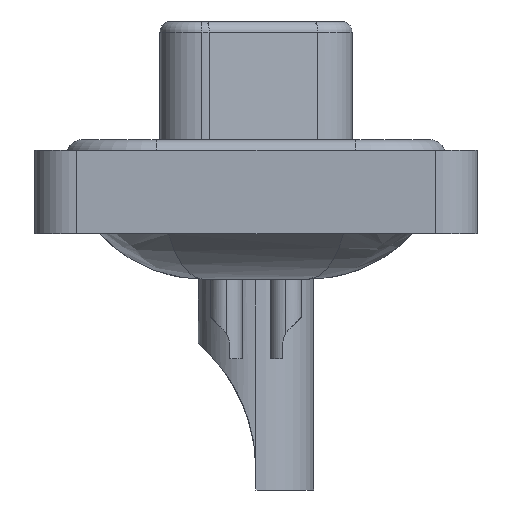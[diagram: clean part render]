
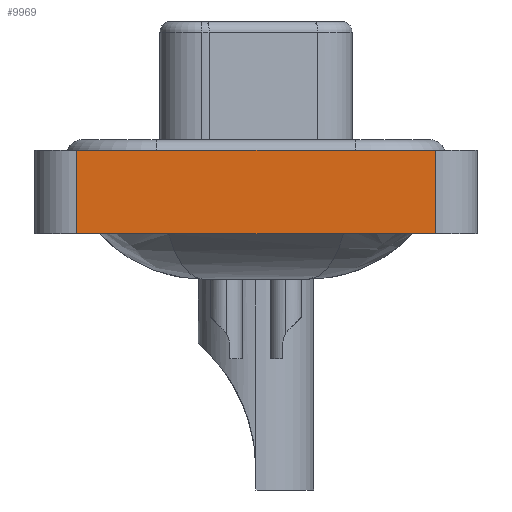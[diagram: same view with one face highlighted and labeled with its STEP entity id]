
A CAD part, left-side view. The second image highlights one B-rep face of the part: STEP entity #9969.
In plain terms, the highlighted planar face has unit normal (-1, 0, 0).
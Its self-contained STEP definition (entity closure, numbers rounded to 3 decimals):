
#1512 = CARTESIAN_POINT ( 'NONE',  ( -7.35, -8.55, -3.6 ) ) ;
#1680 = EDGE_CURVE ( 'NONE', #20873, #17307, #14497, .T. ) ;
#1867 = DIRECTION ( 'NONE',  ( -1., 0., 0. ) ) ;
#1883 = LINE ( 'NONE', #1512, #20298 ) ;
#2558 = ORIENTED_EDGE ( 'NONE', *, *, #10255, .T. ) ;
#2963 = CARTESIAN_POINT ( 'NONE',  ( -7.35, -8.55, -3.6 ) ) ;
#3530 = VECTOR ( 'NONE', #10609, 1000. ) ;
#4002 = PLANE ( 'NONE',  #15526 ) ;
#4175 = VECTOR ( 'NONE', #16267, 1000. ) ;
#6717 = LINE ( 'NONE', #2963, #3530 ) ;
#6854 = DIRECTION ( 'NONE',  ( 0., -1., 0. ) ) ;
#7087 = EDGE_LOOP ( 'NONE', ( #19540, #9354, #21882, #2558 ) ) ;
#7656 = FACE_OUTER_BOUND ( 'NONE', #7087, .T. ) ;
#8632 = CARTESIAN_POINT ( 'NONE',  ( -7.35, 8.55, -3.6 ) ) ;
#8835 = CARTESIAN_POINT ( 'NONE',  ( -7.35, -8.55, -3.6 ) ) ;
#8847 = CARTESIAN_POINT ( 'NONE',  ( -7.35, -8.55, 0.4 ) ) ;
#9354 = ORIENTED_EDGE ( 'NONE', *, *, #1680, .F. ) ;
#9408 = CARTESIAN_POINT ( 'NONE',  ( -7.35, -8.55, -3.6 ) ) ;
#9674 = DIRECTION ( 'NONE',  ( 0., 0., 1. ) ) ;
#9969 = ADVANCED_FACE ( 'NONE', ( #7656 ), #4002, .T. ) ;
#10255 = EDGE_CURVE ( 'NONE', #21236, #19488, #6717, .T. ) ;
#10609 = DIRECTION ( 'NONE',  ( 0., -1., 0. ) ) ;
#11763 = CARTESIAN_POINT ( 'NONE',  ( -7.35, -8.55, 0.4 ) ) ;
#12268 = LINE ( 'NONE', #8632, #4175 ) ;
#14103 = CARTESIAN_POINT ( 'NONE',  ( -7.35, 8.55, 0.4 ) ) ;
#14497 = LINE ( 'NONE', #8847, #17655 ) ;
#15280 = DIRECTION ( 'NONE',  ( 0., 0., 1. ) ) ;
#15526 = AXIS2_PLACEMENT_3D ( 'NONE', #9408, #1867, #15280 ) ;
#16267 = DIRECTION ( 'NONE',  ( 0., 0., 1. ) ) ;
#16982 = EDGE_CURVE ( 'NONE', #19488, #17307, #1883, .T. ) ;
#17307 = VERTEX_POINT ( 'NONE', #11763 ) ;
#17655 = VECTOR ( 'NONE', #6854, 1000. ) ;
#18836 = EDGE_CURVE ( 'NONE', #21236, #20873, #12268, .T. ) ;
#19488 = VERTEX_POINT ( 'NONE', #8835 ) ;
#19540 = ORIENTED_EDGE ( 'NONE', *, *, #16982, .T. ) ;
#20298 = VECTOR ( 'NONE', #9674, 1000. ) ;
#20873 = VERTEX_POINT ( 'NONE', #14103 ) ;
#21236 = VERTEX_POINT ( 'NONE', #23373 ) ;
#21882 = ORIENTED_EDGE ( 'NONE', *, *, #18836, .F. ) ;
#23373 = CARTESIAN_POINT ( 'NONE',  ( -7.35, 8.55, -3.6 ) ) ;
